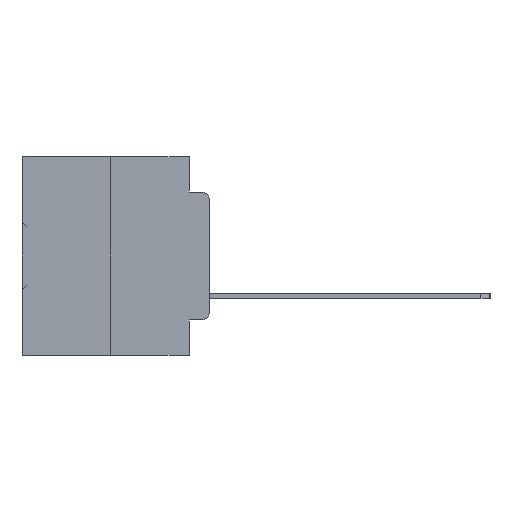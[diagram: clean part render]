
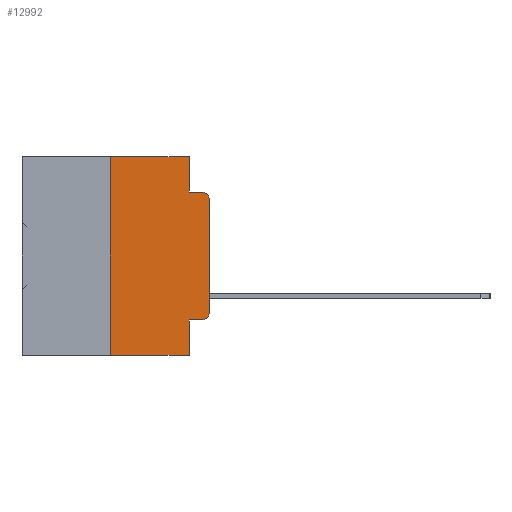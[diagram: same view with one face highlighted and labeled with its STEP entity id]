
A CAD part, left-side view. The second image highlights one B-rep face of the part: STEP entity #12992.
In plain terms, the highlighted planar face has unit normal (-1, 0, 0).
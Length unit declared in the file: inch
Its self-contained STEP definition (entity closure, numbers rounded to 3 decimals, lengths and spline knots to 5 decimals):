
#761 = EDGE_CURVE ( 'NONE', #15867, #16749, #2946, .T. ) ;
#1191 = ORIENTED_EDGE ( 'NONE', *, *, #4018, .F. ) ;
#1292 = EDGE_CURVE ( 'NONE', #31416, #24031, #3850, .T. ) ;
#1700 = LINE ( 'NONE', #24207, #16391 ) ;
#2946 = LINE ( 'NONE', #6279, #32855 ) ;
#3038 = CIRCLE ( 'NONE', #37229, 0.02 ) ;
#3039 = ORIENTED_EDGE ( 'NONE', *, *, #8945, .F. ) ;
#3076 = FACE_OUTER_BOUND ( 'NONE', #36452, .T. ) ;
#3619 = CARTESIAN_POINT ( 'NONE',  ( 0., 0.25, 0. ) ) ;
#3850 = CIRCLE ( 'NONE', #10188, 0.02 ) ;
#3986 = ORIENTED_EDGE ( 'NONE', *, *, #33138, .T. ) ;
#4018 = EDGE_CURVE ( 'NONE', #23858, #35107, #19694, .T. ) ;
#4396 = LINE ( 'NONE', #8237, #25778 ) ;
#4584 = DIRECTION ( 'NONE',  ( 0., 0., -1. ) ) ;
#6279 = CARTESIAN_POINT ( 'NONE',  ( 0., 0.051, -0.4115 ) ) ;
#6290 = DIRECTION ( 'NONE',  ( 0., -1., 0. ) ) ;
#6493 = DIRECTION ( 'NONE',  ( -1., 0., 0. ) ) ;
#6721 = CARTESIAN_POINT ( 'NONE',  ( 0., 0.473, -0.5 ) ) ;
#7314 = ORIENTED_EDGE ( 'NONE', *, *, #29312, .F. ) ;
#7585 = LINE ( 'NONE', #17674, #15250 ) ;
#8237 = CARTESIAN_POINT ( 'NONE',  ( 0., 0.25, 0. ) ) ;
#8945 = EDGE_CURVE ( 'NONE', #9279, #23858, #32162, .T. ) ;
#9279 = VERTEX_POINT ( 'NONE', #3619 ) ;
#9453 = CARTESIAN_POINT ( 'NONE',  ( 0., 0.051, -0.4115 ) ) ;
#10070 = DIRECTION ( 'NONE',  ( -1., 0., 0. ) ) ;
#10188 = AXIS2_PLACEMENT_3D ( 'NONE', #23859, #6493, #26744 ) ;
#10869 = DIRECTION ( 'NONE',  ( 1., 0., 0. ) ) ;
#11150 = DIRECTION ( 'NONE',  ( 0., 0., 1. ) ) ;
#12690 = CARTESIAN_POINT ( 'NONE',  ( 0., 0., -0.1085 ) ) ;
#12992 = ADVANCED_FACE ( 'NONE', ( #3076 ), #28114, .F. ) ;
#13411 = EDGE_CURVE ( 'NONE', #16749, #21169, #3038, .T. ) ;
#13653 = CARTESIAN_POINT ( 'NONE',  ( 0., 0.473, 0. ) ) ;
#15028 = AXIS2_PLACEMENT_3D ( 'NONE', #13653, #10869, #30953 ) ;
#15250 = VECTOR ( 'NONE', #37404, 39.37008 ) ;
#15867 = VERTEX_POINT ( 'NONE', #9453 ) ;
#15982 = CARTESIAN_POINT ( 'NONE',  ( 0., 0.25, -0.5 ) ) ;
#16094 = VECTOR ( 'NONE', #24133, 39.37008 ) ;
#16358 = CARTESIAN_POINT ( 'NONE',  ( 0., 0.051, 0. ) ) ;
#16369 = ORIENTED_EDGE ( 'NONE', *, *, #761, .T. ) ;
#16391 = VECTOR ( 'NONE', #27076, 39.37008 ) ;
#16423 = CARTESIAN_POINT ( 'NONE',  ( 0., 0.051, -0.5 ) ) ;
#16749 = VERTEX_POINT ( 'NONE', #19341 ) ;
#17030 = EDGE_CURVE ( 'NONE', #21169, #31416, #37041, .T. ) ;
#17674 = CARTESIAN_POINT ( 'NONE',  ( 0., 0.051, -0.0885 ) ) ;
#18323 = CARTESIAN_POINT ( 'NONE',  ( 0., 0., 0. ) ) ;
#19341 = CARTESIAN_POINT ( 'NONE',  ( 0., 0.02, -0.4115 ) ) ;
#19694 = LINE ( 'NONE', #16358, #33985 ) ;
#19959 = ORIENTED_EDGE ( 'NONE', *, *, #1292, .T. ) ;
#20045 = CARTESIAN_POINT ( 'NONE',  ( 0., 0.02, -0.0885 ) ) ;
#21169 = VERTEX_POINT ( 'NONE', #26747 ) ;
#23858 = VERTEX_POINT ( 'NONE', #33798 ) ;
#23859 = CARTESIAN_POINT ( 'NONE',  ( 0., 0.02, -0.1085 ) ) ;
#24031 = VERTEX_POINT ( 'NONE', #20045 ) ;
#24080 = DIRECTION ( 'NONE',  ( 0., -1., 0. ) ) ;
#24133 = DIRECTION ( 'NONE',  ( 0., 0., 1. ) ) ;
#24207 = CARTESIAN_POINT ( 'NONE',  ( 0., 0.051, 0. ) ) ;
#24271 = EDGE_CURVE ( 'NONE', #15867, #26063, #1700, .T. ) ;
#25435 = DIRECTION ( 'NONE',  ( 0., -1., 0. ) ) ;
#25511 = VECTOR ( 'NONE', #25435, 39.37008 ) ;
#25778 = VECTOR ( 'NONE', #11150, 39.37008 ) ;
#26063 = VERTEX_POINT ( 'NONE', #16423 ) ;
#26177 = EDGE_CURVE ( 'NONE', #35512, #9279, #4396, .T. ) ;
#26268 = ORIENTED_EDGE ( 'NONE', *, *, #26177, .F. ) ;
#26744 = DIRECTION ( 'NONE',  ( 0., 0., -1. ) ) ;
#26747 = CARTESIAN_POINT ( 'NONE',  ( 0., 0., -0.3915 ) ) ;
#26830 = VECTOR ( 'NONE', #24080, 39.37008 ) ;
#27076 = DIRECTION ( 'NONE',  ( 0., 0., -1. ) ) ;
#27303 = CARTESIAN_POINT ( 'NONE',  ( 0., 0.02, -0.3915 ) ) ;
#28096 = ORIENTED_EDGE ( 'NONE', *, *, #24271, .F. ) ;
#28114 = PLANE ( 'NONE',  #15028 ) ;
#28525 = CARTESIAN_POINT ( 'NONE',  ( 0., 0.051, -0.0885 ) ) ;
#29312 = EDGE_CURVE ( 'NONE', #35107, #24031, #7585, .T. ) ;
#30163 = DIRECTION ( 'NONE',  ( 0., 0., -1. ) ) ;
#30953 = DIRECTION ( 'NONE',  ( 0., 0., -1. ) ) ;
#31416 = VERTEX_POINT ( 'NONE', #12690 ) ;
#32162 = LINE ( 'NONE', #33846, #25511 ) ;
#32526 = ORIENTED_EDGE ( 'NONE', *, *, #13411, .T. ) ;
#32855 = VECTOR ( 'NONE', #6290, 39.37008 ) ;
#33138 = EDGE_CURVE ( 'NONE', #35512, #26063, #34358, .T. ) ;
#33798 = CARTESIAN_POINT ( 'NONE',  ( 0., 0.051, 0. ) ) ;
#33846 = CARTESIAN_POINT ( 'NONE',  ( 0., 0.473, 0. ) ) ;
#33985 = VECTOR ( 'NONE', #4584, 39.37008 ) ;
#34247 = ORIENTED_EDGE ( 'NONE', *, *, #17030, .T. ) ;
#34358 = LINE ( 'NONE', #6721, #26830 ) ;
#35107 = VERTEX_POINT ( 'NONE', #28525 ) ;
#35512 = VERTEX_POINT ( 'NONE', #15982 ) ;
#36452 = EDGE_LOOP ( 'NONE', ( #34247, #19959, #7314, #1191, #3039, #26268, #3986, #28096, #16369, #32526 ) ) ;
#37041 = LINE ( 'NONE', #18323, #16094 ) ;
#37229 = AXIS2_PLACEMENT_3D ( 'NONE', #27303, #10070, #30163 ) ;
#37404 = DIRECTION ( 'NONE',  ( 0., -1., 0. ) ) ;
